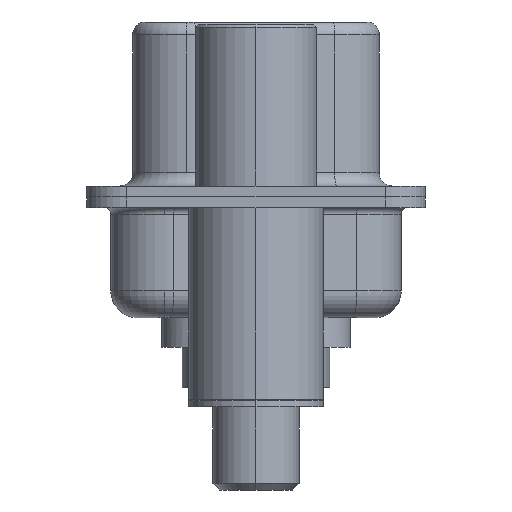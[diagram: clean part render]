
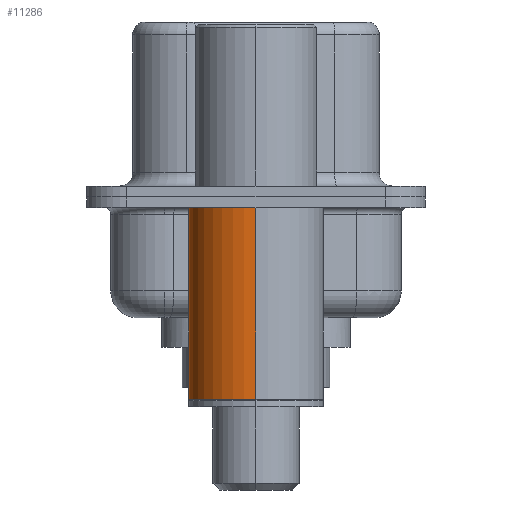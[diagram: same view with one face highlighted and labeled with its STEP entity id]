
A CAD part, left-side view. The second image highlights one B-rep face of the part: STEP entity #11286.
In plain terms, the highlighted cylindrical face has radius 2.5 mm (diameter 5 mm), a partial arc.
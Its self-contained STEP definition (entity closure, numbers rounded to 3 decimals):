
#76 = VERTEX_POINT ( 'NONE', #490 ) ;
#184 = AXIS2_PLACEMENT_3D ( 'NONE', #2064, #12868, #4933 ) ;
#490 = CARTESIAN_POINT ( 'NONE',  ( -2.5, 0., -7.525 ) ) ;
#886 = CARTESIAN_POINT ( 'NONE',  ( 2.5, 0., 0.581 ) ) ;
#1020 = DIRECTION ( 'NONE',  ( 0., 0., 1. ) ) ;
#1542 = CIRCLE ( 'NONE', #2756, 2.5 ) ;
#1616 = DIRECTION ( 'NONE',  ( 0., 0., 1. ) ) ;
#1693 = CARTESIAN_POINT ( 'NONE',  ( 0., 0., -7.525 ) ) ;
#2064 = CARTESIAN_POINT ( 'NONE',  ( 0., 0., 0.581 ) ) ;
#2083 = CIRCLE ( 'NONE', #3223, 2.5 ) ;
#2310 = VERTEX_POINT ( 'NONE', #8146 ) ;
#2429 = EDGE_CURVE ( 'NONE', #11384, #76, #2083, .T. ) ;
#2607 = CARTESIAN_POINT ( 'NONE',  ( -2.5, 0., 0.581 ) ) ;
#2756 = AXIS2_PLACEMENT_3D ( 'NONE', #9795, #1616, #11106 ) ;
#2856 = ORIENTED_EDGE ( 'NONE', *, *, #10931, .F. ) ;
#3223 = AXIS2_PLACEMENT_3D ( 'NONE', #1693, #1020, #5013 ) ;
#4727 = VECTOR ( 'NONE', #16037, 1000. ) ;
#4933 = DIRECTION ( 'NONE',  ( 1., 0., 0. ) ) ;
#5013 = DIRECTION ( 'NONE',  ( 1., 0., 0. ) ) ;
#5059 = VERTEX_POINT ( 'NONE', #9424 ) ;
#5128 = ORIENTED_EDGE ( 'NONE', *, *, #2429, .T. ) ;
#6286 = VECTOR ( 'NONE', #17008, 1000. ) ;
#6953 = EDGE_LOOP ( 'NONE', ( #5128, #13200, #2856, #10571 ) ) ;
#8146 = CARTESIAN_POINT ( 'NONE',  ( -2.5, 0., -0.4 ) ) ;
#8252 = LINE ( 'NONE', #2607, #4727 ) ;
#9186 = CARTESIAN_POINT ( 'NONE',  ( 2.5, 0., -7.525 ) ) ;
#9424 = CARTESIAN_POINT ( 'NONE',  ( 2.5, 0., -0.4 ) ) ;
#9795 = CARTESIAN_POINT ( 'NONE',  ( 0., 0., -0.4 ) ) ;
#10571 = ORIENTED_EDGE ( 'NONE', *, *, #12710, .F. ) ;
#10931 = EDGE_CURVE ( 'NONE', #5059, #2310, #1542, .T. ) ;
#11106 = DIRECTION ( 'NONE',  ( 1., 0., 0. ) ) ;
#11286 = ADVANCED_FACE ( 'NONE', ( #17483 ), #17071, .T. ) ;
#11384 = VERTEX_POINT ( 'NONE', #9186 ) ;
#12710 = EDGE_CURVE ( 'NONE', #11384, #5059, #16008, .T. ) ;
#12868 = DIRECTION ( 'NONE',  ( 0., 0., 1. ) ) ;
#13200 = ORIENTED_EDGE ( 'NONE', *, *, #17126, .T. ) ;
#16008 = LINE ( 'NONE', #886, #6286 ) ;
#16037 = DIRECTION ( 'NONE',  ( 0., 0., 1. ) ) ;
#17008 = DIRECTION ( 'NONE',  ( 0., 0., 1. ) ) ;
#17071 = CYLINDRICAL_SURFACE ( 'NONE', #184, 2.5 ) ;
#17126 = EDGE_CURVE ( 'NONE', #76, #2310, #8252, .T. ) ;
#17483 = FACE_OUTER_BOUND ( 'NONE', #6953, .T. ) ;
